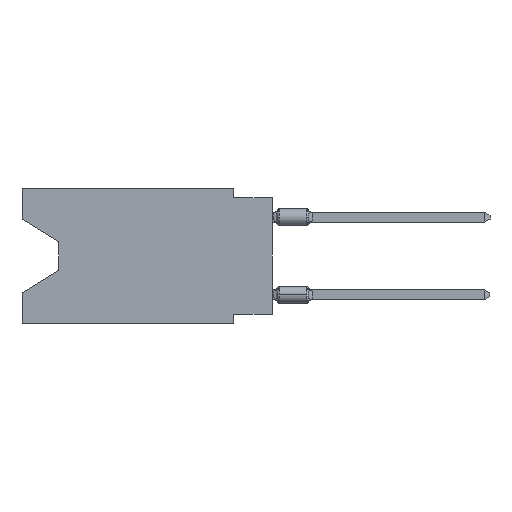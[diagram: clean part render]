
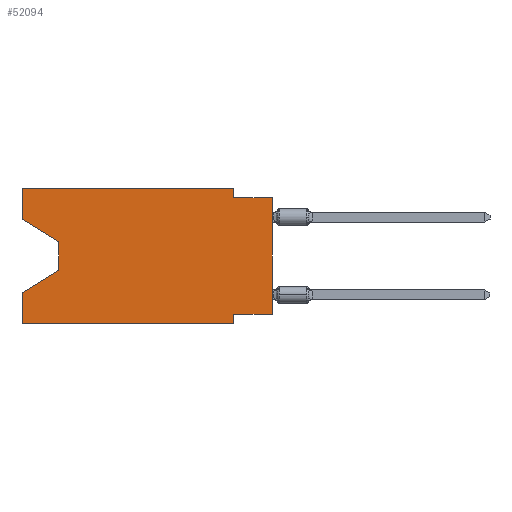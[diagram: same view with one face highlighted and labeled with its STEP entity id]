
A CAD part, left-side view. The second image highlights one B-rep face of the part: STEP entity #52094.
In plain terms, the highlighted planar face has unit normal (-1, 0, 0).
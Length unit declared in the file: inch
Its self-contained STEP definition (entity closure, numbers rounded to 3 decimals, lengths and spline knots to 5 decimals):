
#8 = CARTESIAN_POINT ( 'NONE',  ( 0., 0.55, -0.212 ) ) ;
#289 = VERTEX_POINT ( 'NONE', #12482 ) ;
#406 = VERTEX_POINT ( 'NONE', #44104 ) ;
#680 = LINE ( 'NONE', #36085, #21271 ) ;
#1307 = VECTOR ( 'NONE', #23175, 39.37008 ) ;
#1566 = VERTEX_POINT ( 'NONE', #43959 ) ;
#1671 = VECTOR ( 'NONE', #29706, 39.37008 ) ;
#1748 = EDGE_CURVE ( 'NONE', #51665, #31258, #27862, .T. ) ;
#2344 = ORIENTED_EDGE ( 'NONE', *, *, #12635, .T. ) ;
#2459 = VERTEX_POINT ( 'NONE', #22371 ) ;
#3964 = DIRECTION ( 'NONE',  ( 1., 0., 0. ) ) ;
#4199 = DIRECTION ( 'NONE',  ( 0., -1., 0. ) ) ;
#4484 = CARTESIAN_POINT ( 'NONE',  ( 0., 0.645, 0. ) ) ;
#5669 = DIRECTION ( 'NONE',  ( 0., 1., 0. ) ) ;
#5967 = CARTESIAN_POINT ( 'NONE',  ( 0., 0., -0.025 ) ) ;
#6123 = EDGE_CURVE ( 'NONE', #31258, #289, #15626, .T. ) ;
#6856 = DIRECTION ( 'NONE',  ( 0., -0.855, -0.519 ) ) ;
#7431 = VERTEX_POINT ( 'NONE', #22394 ) ;
#7575 = EDGE_CURVE ( 'NONE', #55311, #50014, #25293, .T. ) ;
#8096 = EDGE_CURVE ( 'NONE', #35601, #2459, #12598, .T. ) ;
#8186 = CARTESIAN_POINT ( 'NONE',  ( 0., 0.645, 0. ) ) ;
#9697 = CARTESIAN_POINT ( 'NONE',  ( 0., 0.1, 0. ) ) ;
#11415 = VECTOR ( 'NONE', #5669, 39.37008 ) ;
#11849 = LINE ( 'NONE', #29980, #1671 ) ;
#12482 = CARTESIAN_POINT ( 'NONE',  ( 0., 0., -0.025 ) ) ;
#12598 = LINE ( 'NONE', #8186, #47082 ) ;
#12635 = EDGE_CURVE ( 'NONE', #406, #289, #32535, .T. ) ;
#13055 = ORIENTED_EDGE ( 'NONE', *, *, #28250, .T. ) ;
#14126 = DIRECTION ( 'NONE',  ( 0., 0., 1. ) ) ;
#14401 = ORIENTED_EDGE ( 'NONE', *, *, #43363, .F. ) ;
#14673 = CARTESIAN_POINT ( 'NONE',  ( 0., 0., 0. ) ) ;
#14818 = VECTOR ( 'NONE', #24630, 39.37008 ) ;
#15626 = LINE ( 'NONE', #5967, #55808 ) ;
#15769 = VECTOR ( 'NONE', #36021, 39.37008 ) ;
#15857 = ORIENTED_EDGE ( 'NONE', *, *, #44661, .F. ) ;
#16601 = LINE ( 'NONE', #34727, #49909 ) ;
#16681 = VECTOR ( 'NONE', #4199, 39.37008 ) ;
#17577 = DIRECTION ( 'NONE',  ( 0., 0., 1. ) ) ;
#18864 = DIRECTION ( 'NONE',  ( 0., -1., 0. ) ) ;
#21271 = VECTOR ( 'NONE', #14126, 39.37008 ) ;
#22267 = CARTESIAN_POINT ( 'NONE',  ( 0., 0.645, -0.35 ) ) ;
#22371 = CARTESIAN_POINT ( 'NONE',  ( 0., 0.645, 0. ) ) ;
#22394 = CARTESIAN_POINT ( 'NONE',  ( 0., 0.645, -0.35 ) ) ;
#23175 = DIRECTION ( 'NONE',  ( 0., 0., -1. ) ) ;
#24317 = VERTEX_POINT ( 'NONE', #45024 ) ;
#24630 = DIRECTION ( 'NONE',  ( 0., 0., 1. ) ) ;
#24928 = AXIS2_PLACEMENT_3D ( 'NONE', #52863, #3964, #56988 ) ;
#25293 = LINE ( 'NONE', #55778, #52611 ) ;
#26763 = LINE ( 'NONE', #4484, #16681 ) ;
#27170 = CARTESIAN_POINT ( 'NONE',  ( 0., 0.1, 0. ) ) ;
#27862 = LINE ( 'NONE', #9697, #1307 ) ;
#28120 = ORIENTED_EDGE ( 'NONE', *, *, #45506, .F. ) ;
#28250 = EDGE_CURVE ( 'NONE', #35601, #55311, #33513, .T. ) ;
#28732 = CARTESIAN_POINT ( 'NONE',  ( 0., 0.645, -0.26975 ) ) ;
#29706 = DIRECTION ( 'NONE',  ( 0., 0., -1. ) ) ;
#29980 = CARTESIAN_POINT ( 'NONE',  ( 0., 0.1, -0.35 ) ) ;
#30862 = LINE ( 'NONE', #57814, #11415 ) ;
#31258 = VERTEX_POINT ( 'NONE', #49898 ) ;
#31364 = EDGE_CURVE ( 'NONE', #406, #1566, #30862, .T. ) ;
#32535 = LINE ( 'NONE', #14673, #14818 ) ;
#33513 = LINE ( 'NONE', #46980, #53238 ) ;
#34105 = ORIENTED_EDGE ( 'NONE', *, *, #7575, .T. ) ;
#34450 = DIRECTION ( 'NONE',  ( 0., 0.855, -0.519 ) ) ;
#34727 = CARTESIAN_POINT ( 'NONE',  ( 0., 0.55, -0.212 ) ) ;
#35601 = VERTEX_POINT ( 'NONE', #39031 ) ;
#36021 = DIRECTION ( 'NONE',  ( 0., -1., 0. ) ) ;
#36085 = CARTESIAN_POINT ( 'NONE',  ( 0., 0.645, 0. ) ) ;
#36389 = EDGE_CURVE ( 'NONE', #50014, #47318, #16601, .T. ) ;
#39031 = CARTESIAN_POINT ( 'NONE',  ( 0., 0.645, -0.08025 ) ) ;
#39684 = FACE_OUTER_BOUND ( 'NONE', #51568, .T. ) ;
#40524 = ORIENTED_EDGE ( 'NONE', *, *, #31364, .F. ) ;
#40787 = ORIENTED_EDGE ( 'NONE', *, *, #54458, .T. ) ;
#42284 = DIRECTION ( 'NONE',  ( 0., 0., -1. ) ) ;
#43363 = EDGE_CURVE ( 'NONE', #1566, #24317, #11849, .T. ) ;
#43959 = CARTESIAN_POINT ( 'NONE',  ( 0., 0.1, -0.325 ) ) ;
#44104 = CARTESIAN_POINT ( 'NONE',  ( 0., 0., -0.325 ) ) ;
#44661 = EDGE_CURVE ( 'NONE', #7431, #47318, #680, .T. ) ;
#44892 = CARTESIAN_POINT ( 'NONE',  ( 0., 0.55, -0.138 ) ) ;
#45024 = CARTESIAN_POINT ( 'NONE',  ( 0., 0.1, -0.35 ) ) ;
#45506 = EDGE_CURVE ( 'NONE', #2459, #51665, #26763, .T. ) ;
#46030 = ORIENTED_EDGE ( 'NONE', *, *, #36389, .T. ) ;
#46980 = CARTESIAN_POINT ( 'NONE',  ( 0., 0.645, -0.08025 ) ) ;
#47082 = VECTOR ( 'NONE', #17577, 39.37008 ) ;
#47209 = ORIENTED_EDGE ( 'NONE', *, *, #1748, .F. ) ;
#47318 = VERTEX_POINT ( 'NONE', #28732 ) ;
#49898 = CARTESIAN_POINT ( 'NONE',  ( 0., 0.1, -0.025 ) ) ;
#49909 = VECTOR ( 'NONE', #34450, 39.37008 ) ;
#50014 = VERTEX_POINT ( 'NONE', #8 ) ;
#50829 = ORIENTED_EDGE ( 'NONE', *, *, #6123, .F. ) ;
#51568 = EDGE_LOOP ( 'NONE', ( #13055, #34105, #46030, #15857, #40787, #14401, #40524, #2344, #50829, #47209, #28120, #55320 ) ) ;
#51665 = VERTEX_POINT ( 'NONE', #27170 ) ;
#52094 = ADVANCED_FACE ( 'NONE', ( #39684 ), #57568, .F. ) ;
#52611 = VECTOR ( 'NONE', #42284, 39.37008 ) ;
#52863 = CARTESIAN_POINT ( 'NONE',  ( 0., 0.645, 0. ) ) ;
#53005 = LINE ( 'NONE', #22267, #15769 ) ;
#53238 = VECTOR ( 'NONE', #6856, 39.37008 ) ;
#54458 = EDGE_CURVE ( 'NONE', #7431, #24317, #53005, .T. ) ;
#55311 = VERTEX_POINT ( 'NONE', #44892 ) ;
#55320 = ORIENTED_EDGE ( 'NONE', *, *, #8096, .F. ) ;
#55778 = CARTESIAN_POINT ( 'NONE',  ( 0., 0.55, -0.138 ) ) ;
#55808 = VECTOR ( 'NONE', #18864, 39.37008 ) ;
#56988 = DIRECTION ( 'NONE',  ( 0., 0., -1. ) ) ;
#57568 = PLANE ( 'NONE',  #24928 ) ;
#57814 = CARTESIAN_POINT ( 'NONE',  ( 0., 0., -0.325 ) ) ;
